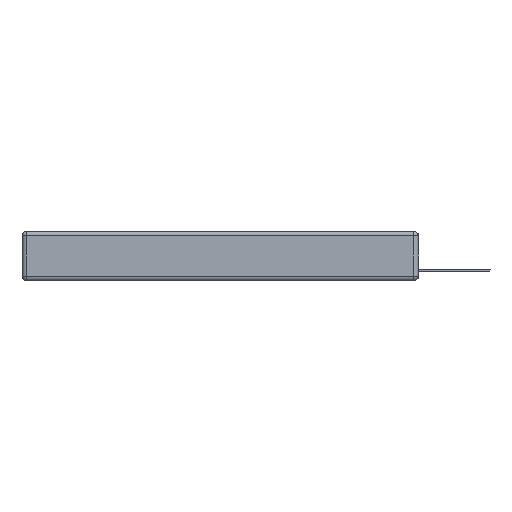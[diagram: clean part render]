
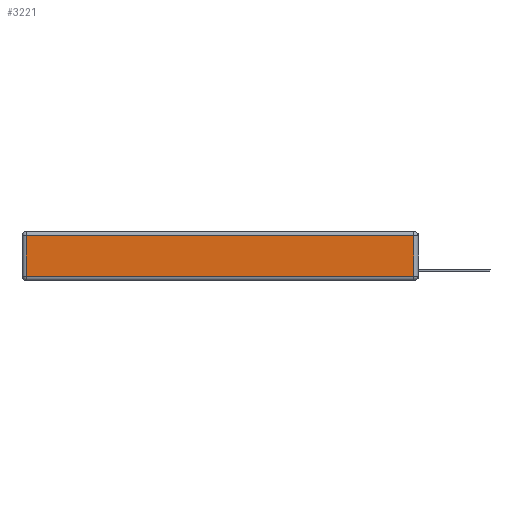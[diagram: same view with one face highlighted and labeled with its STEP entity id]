
A CAD part, left-side view. The second image highlights one B-rep face of the part: STEP entity #3221.
In plain terms, the highlighted planar face has unit normal (-1, 0, 0).
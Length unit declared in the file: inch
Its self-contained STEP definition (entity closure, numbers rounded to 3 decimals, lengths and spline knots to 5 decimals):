
#467 = VECTOR ( 'NONE', #10363, 39.37008 ) ;
#686 = CARTESIAN_POINT ( 'NONE',  ( 0., 2.72, -0.03 ) ) ;
#989 = CARTESIAN_POINT ( 'NONE',  ( 0., 2.72, -0.313 ) ) ;
#1271 = ORIENTED_EDGE ( 'NONE', *, *, #3906, .T. ) ;
#1516 = ORIENTED_EDGE ( 'NONE', *, *, #21619, .T. ) ;
#1529 = LINE ( 'NONE', #14811, #8172 ) ;
#2151 = CARTESIAN_POINT ( 'NONE',  ( 0., 2.75, -0.03 ) ) ;
#3221 = ADVANCED_FACE ( 'NONE', ( #7715 ), #8035, .T. ) ;
#3359 = ORIENTED_EDGE ( 'NONE', *, *, #19736, .T. ) ;
#3902 = LINE ( 'NONE', #11997, #7345 ) ;
#3906 = EDGE_CURVE ( 'NONE', #12040, #10841, #3902, .T. ) ;
#4680 = LINE ( 'NONE', #6219, #13432 ) ;
#6219 = CARTESIAN_POINT ( 'NONE',  ( 0., 2.72, -0.343 ) ) ;
#7345 = VECTOR ( 'NONE', #13986, 39.37008 ) ;
#7715 = FACE_OUTER_BOUND ( 'NONE', #14007, .T. ) ;
#8035 = PLANE ( 'NONE',  #11302 ) ;
#8073 = VERTEX_POINT ( 'NONE', #11349 ) ;
#8172 = VECTOR ( 'NONE', #21451, 39.37008 ) ;
#8316 = DIRECTION ( 'NONE',  ( 0., 0., -1. ) ) ;
#8419 = CARTESIAN_POINT ( 'NONE',  ( 0., 0.03, -0.313 ) ) ;
#9035 = ORIENTED_EDGE ( 'NONE', *, *, #10877, .T. ) ;
#10363 = DIRECTION ( 'NONE',  ( 0., 1., 0. ) ) ;
#10841 = VERTEX_POINT ( 'NONE', #8419 ) ;
#10877 = EDGE_CURVE ( 'NONE', #18940, #12040, #4680, .T. ) ;
#11302 = AXIS2_PLACEMENT_3D ( 'NONE', #12935, #14461, #16236 ) ;
#11349 = CARTESIAN_POINT ( 'NONE',  ( 0., 0.03, -0.03 ) ) ;
#11997 = CARTESIAN_POINT ( 'NONE',  ( 0., 0., -0.313 ) ) ;
#12040 = VERTEX_POINT ( 'NONE', #989 ) ;
#12935 = CARTESIAN_POINT ( 'NONE',  ( 0., 0., -0.343 ) ) ;
#13432 = VECTOR ( 'NONE', #8316, 39.37008 ) ;
#13904 = LINE ( 'NONE', #2151, #467 ) ;
#13986 = DIRECTION ( 'NONE',  ( 0., -1., 0. ) ) ;
#14007 = EDGE_LOOP ( 'NONE', ( #1271, #3359, #1516, #9035 ) ) ;
#14461 = DIRECTION ( 'NONE',  ( -1., 0., 0. ) ) ;
#14811 = CARTESIAN_POINT ( 'NONE',  ( 0., 0.03, -0.343 ) ) ;
#16236 = DIRECTION ( 'NONE',  ( 0., 0., 1. ) ) ;
#18940 = VERTEX_POINT ( 'NONE', #686 ) ;
#19736 = EDGE_CURVE ( 'NONE', #10841, #8073, #1529, .T. ) ;
#21451 = DIRECTION ( 'NONE',  ( 0., 0., 1. ) ) ;
#21619 = EDGE_CURVE ( 'NONE', #8073, #18940, #13904, .T. ) ;
